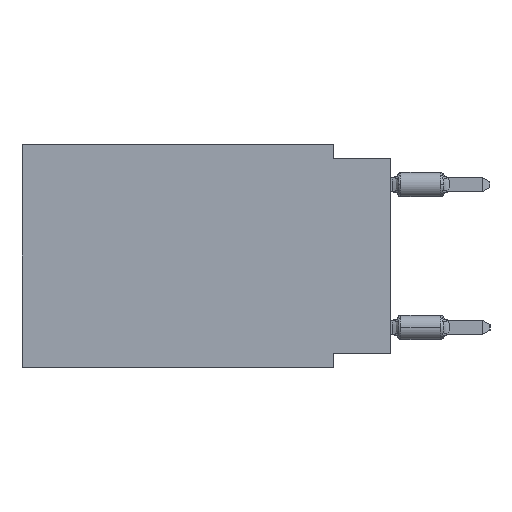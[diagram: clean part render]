
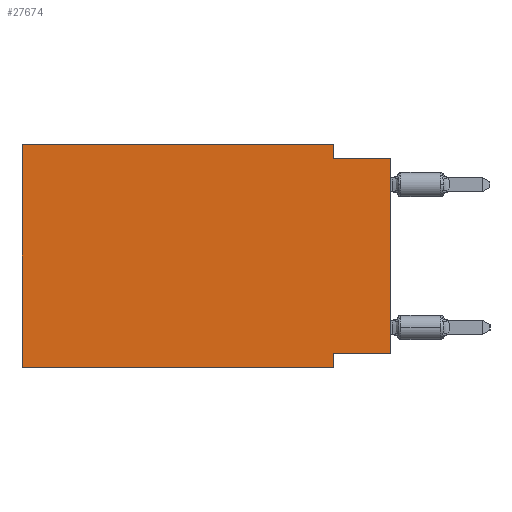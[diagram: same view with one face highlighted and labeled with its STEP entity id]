
A CAD part, left-side view. The second image highlights one B-rep face of the part: STEP entity #27674.
In plain terms, the highlighted planar face has unit normal (-1, 0, 0).
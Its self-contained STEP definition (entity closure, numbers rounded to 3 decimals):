
#1796 = CARTESIAN_POINT ( 'NONE',  ( 0., 16.383, 0. ) ) ;
#2552 = VECTOR ( 'NONE', #20056, 1000. ) ;
#3472 = ORIENTED_EDGE ( 'NONE', *, *, #28745, .F. ) ;
#4678 = VECTOR ( 'NONE', #48733, 1000. ) ;
#5380 = LINE ( 'NONE', #14963, #10374 ) ;
#6288 = FACE_OUTER_BOUND ( 'NONE', #58155, .T. ) ;
#7245 = VECTOR ( 'NONE', #15377, 1000. ) ;
#7331 = LINE ( 'NONE', #48676, #51694 ) ;
#9216 = CARTESIAN_POINT ( 'NONE',  ( 0., 0., 0. ) ) ;
#10374 = VECTOR ( 'NONE', #46730, 1000. ) ;
#12065 = VECTOR ( 'NONE', #37220, 1000. ) ;
#12749 = LINE ( 'NONE', #45957, #40393 ) ;
#12981 = VERTEX_POINT ( 'NONE', #49886 ) ;
#14001 = EDGE_CURVE ( 'NONE', #45664, #19955, #34372, .T. ) ;
#14963 = CARTESIAN_POINT ( 'NONE',  ( 0., 0., -9.271 ) ) ;
#15377 = DIRECTION ( 'NONE',  ( 0., 0., -1. ) ) ;
#15572 = DIRECTION ( 'NONE',  ( 1., 0., 0. ) ) ;
#15595 = CARTESIAN_POINT ( 'NONE',  ( 0., 2.54, -9.906 ) ) ;
#18773 = AXIS2_PLACEMENT_3D ( 'NONE', #1796, #15572, #33864 ) ;
#18956 = VERTEX_POINT ( 'NONE', #44837 ) ;
#19552 = LINE ( 'NONE', #24038, #12065 ) ;
#19955 = VERTEX_POINT ( 'NONE', #34389 ) ;
#20056 = DIRECTION ( 'NONE',  ( 0., 0., -1. ) ) ;
#21121 = DIRECTION ( 'NONE',  ( 0., 0., 1. ) ) ;
#21284 = ORIENTED_EDGE ( 'NONE', *, *, #14001, .F. ) ;
#21950 = EDGE_CURVE ( 'NONE', #26341, #58332, #56425, .T. ) ;
#22504 = EDGE_CURVE ( 'NONE', #12981, #23845, #19552, .T. ) ;
#23845 = VERTEX_POINT ( 'NONE', #51615 ) ;
#23879 = CARTESIAN_POINT ( 'NONE',  ( 0., 16.383, 0. ) ) ;
#24038 = CARTESIAN_POINT ( 'NONE',  ( 0., 0., -0.635 ) ) ;
#24564 = PLANE ( 'NONE',  #18773 ) ;
#26341 = VERTEX_POINT ( 'NONE', #52929 ) ;
#27674 = ADVANCED_FACE ( 'NONE', ( #6288 ), #24564, .F. ) ;
#27842 = CARTESIAN_POINT ( 'NONE',  ( 0., 2.54, 0. ) ) ;
#27852 = CARTESIAN_POINT ( 'NONE',  ( 0., 16.383, -9.906 ) ) ;
#27861 = EDGE_CURVE ( 'NONE', #18956, #23845, #46048, .T. ) ;
#28010 = ORIENTED_EDGE ( 'NONE', *, *, #38351, .T. ) ;
#28745 = EDGE_CURVE ( 'NONE', #18956, #26341, #5380, .T. ) ;
#31349 = EDGE_CURVE ( 'NONE', #45323, #45664, #7331, .T. ) ;
#33864 = DIRECTION ( 'NONE',  ( 0., 0., -1. ) ) ;
#34372 = LINE ( 'NONE', #49022, #4678 ) ;
#34389 = CARTESIAN_POINT ( 'NONE',  ( 0., 2.54, 0. ) ) ;
#37220 = DIRECTION ( 'NONE',  ( 0., -1., 0. ) ) ;
#38351 = EDGE_CURVE ( 'NONE', #45323, #58332, #12749, .T. ) ;
#40393 = VECTOR ( 'NONE', #54669, 1000. ) ;
#42153 = ORIENTED_EDGE ( 'NONE', *, *, #31349, .F. ) ;
#42365 = ORIENTED_EDGE ( 'NONE', *, *, #22504, .F. ) ;
#44075 = ORIENTED_EDGE ( 'NONE', *, *, #27861, .T. ) ;
#44837 = CARTESIAN_POINT ( 'NONE',  ( 0., 0., -9.271 ) ) ;
#45323 = VERTEX_POINT ( 'NONE', #27852 ) ;
#45664 = VERTEX_POINT ( 'NONE', #23879 ) ;
#45957 = CARTESIAN_POINT ( 'NONE',  ( 0., 16.383, -9.906 ) ) ;
#46048 = LINE ( 'NONE', #9216, #52286 ) ;
#46408 = ORIENTED_EDGE ( 'NONE', *, *, #21950, .F. ) ;
#46730 = DIRECTION ( 'NONE',  ( 0., 1., 0. ) ) ;
#48030 = CARTESIAN_POINT ( 'NONE',  ( 0., 2.54, -9.906 ) ) ;
#48676 = CARTESIAN_POINT ( 'NONE',  ( 0., 16.383, 0. ) ) ;
#48733 = DIRECTION ( 'NONE',  ( 0., -1., 0. ) ) ;
#49022 = CARTESIAN_POINT ( 'NONE',  ( 0., 16.383, 0. ) ) ;
#49886 = CARTESIAN_POINT ( 'NONE',  ( 0., 2.54, -0.635 ) ) ;
#50736 = ORIENTED_EDGE ( 'NONE', *, *, #56376, .F. ) ;
#51615 = CARTESIAN_POINT ( 'NONE',  ( 0., 0., -0.635 ) ) ;
#51694 = VECTOR ( 'NONE', #21121, 1000. ) ;
#52286 = VECTOR ( 'NONE', #55349, 1000. ) ;
#52929 = CARTESIAN_POINT ( 'NONE',  ( 0., 2.54, -9.271 ) ) ;
#54669 = DIRECTION ( 'NONE',  ( 0., -1., 0. ) ) ;
#55349 = DIRECTION ( 'NONE',  ( 0., 0., 1. ) ) ;
#56298 = LINE ( 'NONE', #27842, #2552 ) ;
#56376 = EDGE_CURVE ( 'NONE', #19955, #12981, #56298, .T. ) ;
#56425 = LINE ( 'NONE', #48030, #7245 ) ;
#58155 = EDGE_LOOP ( 'NONE', ( #44075, #42365, #50736, #21284, #42153, #28010, #46408, #3472 ) ) ;
#58332 = VERTEX_POINT ( 'NONE', #15595 ) ;
